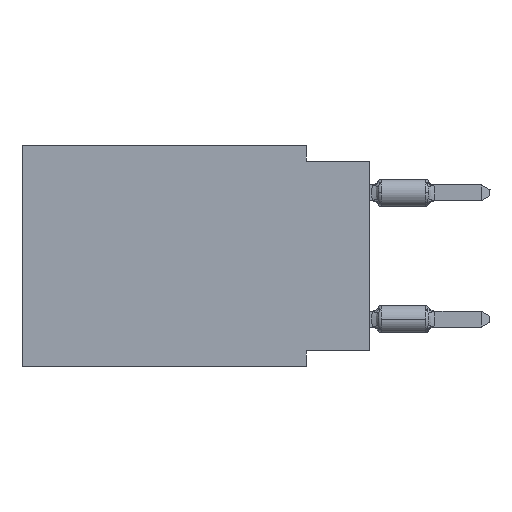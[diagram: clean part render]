
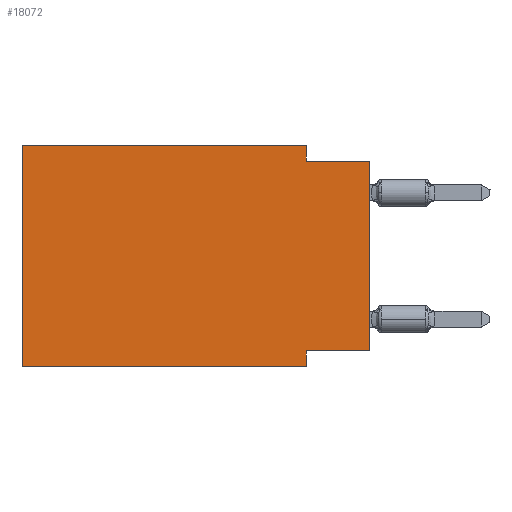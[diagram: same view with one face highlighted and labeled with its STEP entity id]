
A CAD part, left-side view. The second image highlights one B-rep face of the part: STEP entity #18072.
In plain terms, the highlighted planar face has unit normal (-1, 0, 0).
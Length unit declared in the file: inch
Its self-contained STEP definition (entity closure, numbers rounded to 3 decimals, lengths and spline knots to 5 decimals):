
#42 = EDGE_LOOP ( 'NONE', ( #17894, #17477, #8865, #3355, #4849, #1877, #6420, #17652 ) ) ;
#116 = VERTEX_POINT ( 'NONE', #6229 ) ;
#355 = DIRECTION ( 'NONE',  ( 1., 0., 0. ) ) ;
#710 = FACE_OUTER_BOUND ( 'NONE', #42, .T. ) ;
#719 = CARTESIAN_POINT ( 'NONE',  ( 0., 0.1, -0.025 ) ) ;
#965 = CARTESIAN_POINT ( 'NONE',  ( 0., 0.55, -0.35 ) ) ;
#1476 = EDGE_CURVE ( 'NONE', #3375, #1867, #7950, .T. ) ;
#1867 = VERTEX_POINT ( 'NONE', #9067 ) ;
#1868 = LINE ( 'NONE', #4506, #17506 ) ;
#1877 = ORIENTED_EDGE ( 'NONE', *, *, #5939, .T. ) ;
#1961 = DIRECTION ( 'NONE',  ( 0., 0., -1. ) ) ;
#2004 = VECTOR ( 'NONE', #5878, 39.37008 ) ;
#2646 = LINE ( 'NONE', #8312, #6060 ) ;
#3350 = VERTEX_POINT ( 'NONE', #3546 ) ;
#3355 = ORIENTED_EDGE ( 'NONE', *, *, #5031, .F. ) ;
#3375 = VERTEX_POINT ( 'NONE', #719 ) ;
#3546 = CARTESIAN_POINT ( 'NONE',  ( 0., 0., -0.325 ) ) ;
#3916 = CARTESIAN_POINT ( 'NONE',  ( 0., 0., -0.025 ) ) ;
#4452 = PLANE ( 'NONE',  #10517 ) ;
#4506 = CARTESIAN_POINT ( 'NONE',  ( 0., 0.1, -0.35 ) ) ;
#4650 = DIRECTION ( 'NONE',  ( 0., 0., -1. ) ) ;
#4671 = LINE ( 'NONE', #8980, #13123 ) ;
#4738 = EDGE_CURVE ( 'NONE', #3350, #12229, #13757, .T. ) ;
#4849 = ORIENTED_EDGE ( 'NONE', *, *, #13013, .F. ) ;
#5031 = EDGE_CURVE ( 'NONE', #12500, #116, #10605, .T. ) ;
#5878 = DIRECTION ( 'NONE',  ( 0., 0., -1. ) ) ;
#5939 = EDGE_CURVE ( 'NONE', #6459, #12051, #7660, .T. ) ;
#6060 = VECTOR ( 'NONE', #14930, 39.37008 ) ;
#6151 = CARTESIAN_POINT ( 'NONE',  ( 0., 0.1, 0. ) ) ;
#6229 = CARTESIAN_POINT ( 'NONE',  ( 0., 0.1, 0. ) ) ;
#6420 = ORIENTED_EDGE ( 'NONE', *, *, #14156, .F. ) ;
#6459 = VERTEX_POINT ( 'NONE', #9733 ) ;
#7112 = VECTOR ( 'NONE', #9397, 39.37008 ) ;
#7349 = LINE ( 'NONE', #6151, #2004 ) ;
#7660 = LINE ( 'NONE', #965, #7112 ) ;
#7950 = LINE ( 'NONE', #3916, #17699 ) ;
#8091 = CARTESIAN_POINT ( 'NONE',  ( 0., 0.55, 0. ) ) ;
#8312 = CARTESIAN_POINT ( 'NONE',  ( 0., 0., 0. ) ) ;
#8646 = EDGE_CURVE ( 'NONE', #3350, #1867, #2646, .T. ) ;
#8846 = CARTESIAN_POINT ( 'NONE',  ( 0., 0.1, -0.325 ) ) ;
#8865 = ORIENTED_EDGE ( 'NONE', *, *, #9607, .F. ) ;
#8980 = CARTESIAN_POINT ( 'NONE',  ( 0., 0.55, 0. ) ) ;
#9067 = CARTESIAN_POINT ( 'NONE',  ( 0., 0., -0.025 ) ) ;
#9397 = DIRECTION ( 'NONE',  ( 0., -1., 0. ) ) ;
#9607 = EDGE_CURVE ( 'NONE', #116, #3375, #7349, .T. ) ;
#9615 = DIRECTION ( 'NONE',  ( 0., 1., 0. ) ) ;
#9733 = CARTESIAN_POINT ( 'NONE',  ( 0., 0.55, -0.35 ) ) ;
#10174 = DIRECTION ( 'NONE',  ( 0., 0., 1. ) ) ;
#10517 = AXIS2_PLACEMENT_3D ( 'NONE', #17204, #355, #4650 ) ;
#10605 = LINE ( 'NONE', #8091, #14716 ) ;
#11294 = CARTESIAN_POINT ( 'NONE',  ( 0., 0.55, 0. ) ) ;
#12051 = VERTEX_POINT ( 'NONE', #16371 ) ;
#12229 = VERTEX_POINT ( 'NONE', #8846 ) ;
#12500 = VERTEX_POINT ( 'NONE', #11294 ) ;
#13013 = EDGE_CURVE ( 'NONE', #6459, #12500, #4671, .T. ) ;
#13123 = VECTOR ( 'NONE', #10174, 39.37008 ) ;
#13757 = LINE ( 'NONE', #16409, #14217 ) ;
#14156 = EDGE_CURVE ( 'NONE', #12229, #12051, #1868, .T. ) ;
#14217 = VECTOR ( 'NONE', #9615, 39.37008 ) ;
#14716 = VECTOR ( 'NONE', #16201, 39.37008 ) ;
#14930 = DIRECTION ( 'NONE',  ( 0., 0., 1. ) ) ;
#16201 = DIRECTION ( 'NONE',  ( 0., -1., 0. ) ) ;
#16371 = CARTESIAN_POINT ( 'NONE',  ( 0., 0.1, -0.35 ) ) ;
#16409 = CARTESIAN_POINT ( 'NONE',  ( 0., 0., -0.325 ) ) ;
#17204 = CARTESIAN_POINT ( 'NONE',  ( 0., 0.55, 0. ) ) ;
#17477 = ORIENTED_EDGE ( 'NONE', *, *, #1476, .F. ) ;
#17506 = VECTOR ( 'NONE', #1961, 39.37008 ) ;
#17652 = ORIENTED_EDGE ( 'NONE', *, *, #4738, .F. ) ;
#17699 = VECTOR ( 'NONE', #17949, 39.37008 ) ;
#17894 = ORIENTED_EDGE ( 'NONE', *, *, #8646, .T. ) ;
#17949 = DIRECTION ( 'NONE',  ( 0., -1., 0. ) ) ;
#18072 = ADVANCED_FACE ( 'NONE', ( #710 ), #4452, .F. ) ;
